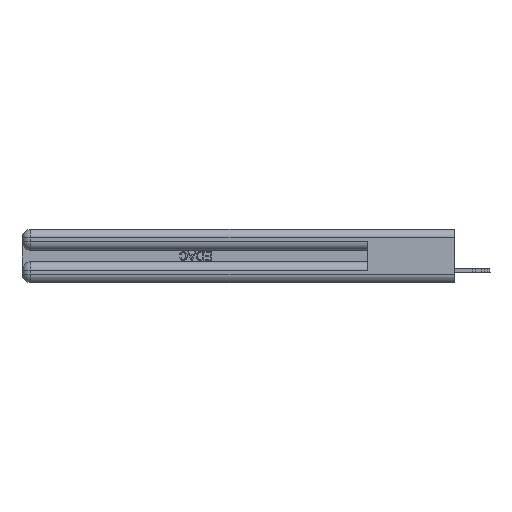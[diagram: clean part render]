
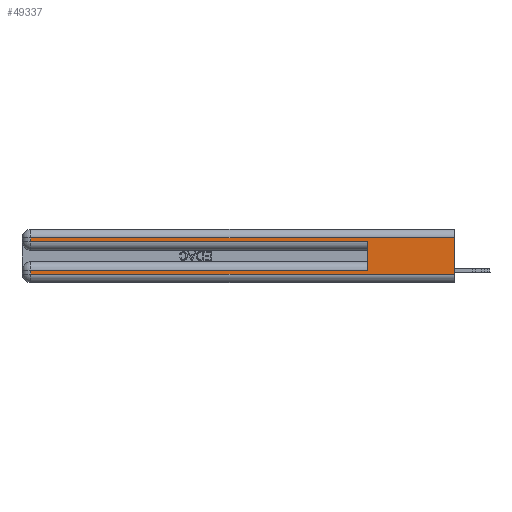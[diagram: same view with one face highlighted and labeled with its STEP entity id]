
A CAD part, left-side view. The second image highlights one B-rep face of the part: STEP entity #49337.
In plain terms, the highlighted planar face has unit normal (-1, 0, 0).
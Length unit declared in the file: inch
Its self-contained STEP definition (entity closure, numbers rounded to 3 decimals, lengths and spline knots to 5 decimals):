
#463 = LINE ( 'NONE', #43010, #46575 ) ;
#1692 = CARTESIAN_POINT ( 'NONE',  ( 0., 2.94, 0.285 ) ) ;
#2464 = VERTEX_POINT ( 'NONE', #17380 ) ;
#3271 = VERTEX_POINT ( 'NONE', #1692 ) ;
#5641 = ORIENTED_EDGE ( 'NONE', *, *, #36540, .T. ) ;
#6081 = CARTESIAN_POINT ( 'NONE',  ( 0., 0., 0.31 ) ) ;
#7294 = DIRECTION ( 'NONE',  ( 0., -1., 0. ) ) ;
#9113 = CARTESIAN_POINT ( 'NONE',  ( 0., 0.6, 0.145 ) ) ;
#9294 = DIRECTION ( 'NONE',  ( 0., -1., 0. ) ) ;
#10910 = CARTESIAN_POINT ( 'NONE',  ( 0., 0., 0.37 ) ) ;
#11086 = DIRECTION ( 'NONE',  ( 0., 0., -1. ) ) ;
#11241 = LINE ( 'NONE', #32087, #47498 ) ;
#11389 = VECTOR ( 'NONE', #23055, 39.37008 ) ;
#12540 = CARTESIAN_POINT ( 'NONE',  ( 0., 0., 0.06 ) ) ;
#12776 = CARTESIAN_POINT ( 'NONE',  ( 0., 0.6, 0.085 ) ) ;
#14149 = DIRECTION ( 'NONE',  ( 0., 0., -1. ) ) ;
#14283 = AXIS2_PLACEMENT_3D ( 'NONE', #10910, #22744, #11086 ) ;
#14795 = EDGE_LOOP ( 'NONE', ( #27119, #5641, #19243, #22613, #28740, #28759, #41788, #35837 ) ) ;
#15796 = LINE ( 'NONE', #48145, #45941 ) ;
#16102 = DIRECTION ( 'NONE',  ( 0., 1., 0. ) ) ;
#16308 = LINE ( 'NONE', #42665, #11389 ) ;
#16412 = EDGE_CURVE ( 'NONE', #21974, #2464, #11241, .T. ) ;
#17059 = LINE ( 'NONE', #17364, #30567 ) ;
#17364 = CARTESIAN_POINT ( 'NONE',  ( 0., 0., 0.06 ) ) ;
#17380 = CARTESIAN_POINT ( 'NONE',  ( 0., 2.94, 0.06 ) ) ;
#19243 = ORIENTED_EDGE ( 'NONE', *, *, #25057, .T. ) ;
#20553 = CARTESIAN_POINT ( 'NONE',  ( 0., 0., 0.31 ) ) ;
#21974 = VERTEX_POINT ( 'NONE', #32454 ) ;
#22613 = ORIENTED_EDGE ( 'NONE', *, *, #22643, .T. ) ;
#22643 = EDGE_CURVE ( 'NONE', #3271, #24382, #463, .T. ) ;
#22744 = DIRECTION ( 'NONE',  ( 1., 0., 0. ) ) ;
#23055 = DIRECTION ( 'NONE',  ( 0., 1., 0. ) ) ;
#23930 = CARTESIAN_POINT ( 'NONE',  ( 0., 0.6, 0.285 ) ) ;
#24382 = VERTEX_POINT ( 'NONE', #23930 ) ;
#24840 = EDGE_CURVE ( 'NONE', #35512, #43038, #15796, .T. ) ;
#25057 = EDGE_CURVE ( 'NONE', #41049, #3271, #31111, .T. ) ;
#26372 = PLANE ( 'NONE',  #14283 ) ;
#26979 = VECTOR ( 'NONE', #16102, 39.37008 ) ;
#27119 = ORIENTED_EDGE ( 'NONE', *, *, #24840, .F. ) ;
#28240 = DIRECTION ( 'NONE',  ( 0., 0., -1. ) ) ;
#28740 = ORIENTED_EDGE ( 'NONE', *, *, #38452, .F. ) ;
#28759 = ORIENTED_EDGE ( 'NONE', *, *, #32639, .T. ) ;
#30567 = VECTOR ( 'NONE', #9294, 39.37008 ) ;
#31111 = LINE ( 'NONE', #45935, #41607 ) ;
#32087 = CARTESIAN_POINT ( 'NONE',  ( 0., 2.94, 0.37 ) ) ;
#32454 = CARTESIAN_POINT ( 'NONE',  ( 0., 2.94, 0.085 ) ) ;
#32545 = CARTESIAN_POINT ( 'NONE',  ( 0., 2.94, 0.31 ) ) ;
#32639 = EDGE_CURVE ( 'NONE', #35433, #21974, #16308, .T. ) ;
#35433 = VERTEX_POINT ( 'NONE', #12776 ) ;
#35512 = VERTEX_POINT ( 'NONE', #6081 ) ;
#35837 = ORIENTED_EDGE ( 'NONE', *, *, #47505, .T. ) ;
#36540 = EDGE_CURVE ( 'NONE', #35512, #41049, #37453, .T. ) ;
#36918 = LINE ( 'NONE', #9113, #42433 ) ;
#37453 = LINE ( 'NONE', #20553, #26979 ) ;
#38452 = EDGE_CURVE ( 'NONE', #35433, #24382, #36918, .T. ) ;
#39082 = FACE_OUTER_BOUND ( 'NONE', #14795, .T. ) ;
#41049 = VERTEX_POINT ( 'NONE', #32545 ) ;
#41607 = VECTOR ( 'NONE', #14149, 39.37008 ) ;
#41788 = ORIENTED_EDGE ( 'NONE', *, *, #16412, .T. ) ;
#42433 = VECTOR ( 'NONE', #44005, 39.37008 ) ;
#42665 = CARTESIAN_POINT ( 'NONE',  ( 0., 0., 0.085 ) ) ;
#43010 = CARTESIAN_POINT ( 'NONE',  ( 0., 0., 0.285 ) ) ;
#43038 = VERTEX_POINT ( 'NONE', #12540 ) ;
#44005 = DIRECTION ( 'NONE',  ( 0., 0., 1. ) ) ;
#45288 = DIRECTION ( 'NONE',  ( 0., 0., -1. ) ) ;
#45935 = CARTESIAN_POINT ( 'NONE',  ( 0., 2.94, 0.37 ) ) ;
#45941 = VECTOR ( 'NONE', #28240, 39.37008 ) ;
#46575 = VECTOR ( 'NONE', #7294, 39.37008 ) ;
#47498 = VECTOR ( 'NONE', #45288, 39.37008 ) ;
#47505 = EDGE_CURVE ( 'NONE', #2464, #43038, #17059, .T. ) ;
#48145 = CARTESIAN_POINT ( 'NONE',  ( 0., 0., 0.37 ) ) ;
#49337 = ADVANCED_FACE ( 'NONE', ( #39082 ), #26372, .F. ) ;
